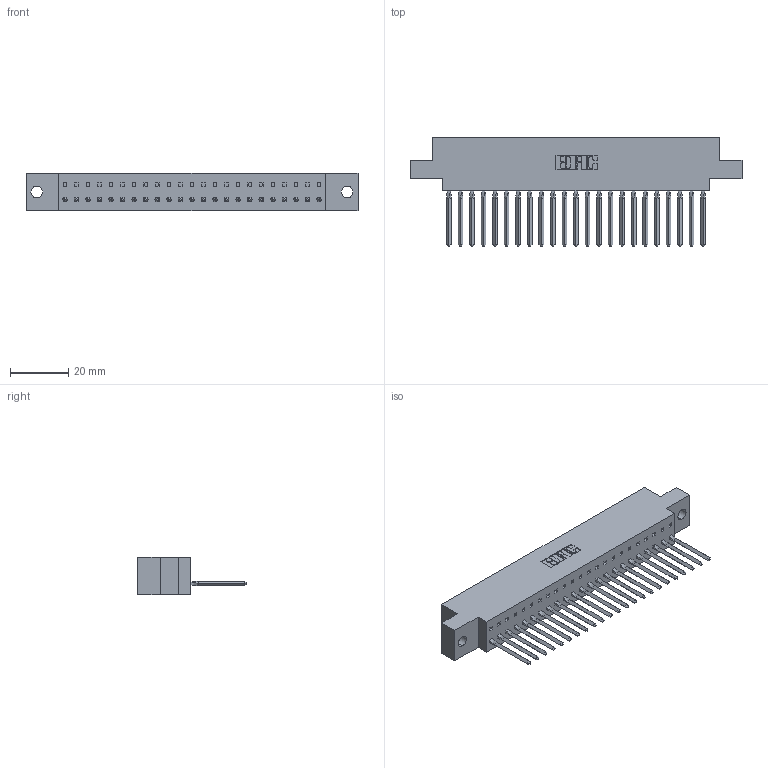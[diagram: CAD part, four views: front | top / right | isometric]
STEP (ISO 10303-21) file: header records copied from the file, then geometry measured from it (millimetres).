
FILE_DESCRIPTION (( 'STEP AP203' ), '1' );
FILE_NAME ('317-023-541-604.STEP', '2020-02-27T17:47:08', ( '' ), ( '' ), 'SwSTEP 2.0', 'SolidWorks 2016', '' );
FILE_SCHEMA (( 'CONFIG_CONTROL_DESIGN' ));
Length unit declared in the file: inch
Products named in the file (3): 317 Part_.156 Dia - TH; 317-290-002_541; 317-023-541-604
Assembly tree (24 placements, depth 2):
  317-023-541-604
    317 Part_.156 Dia - TH
    317-290-002_541  x23
Bounding box: 113.84 x 37.34 x 12.7 mm (x, y, z)
Volume: 17789.4 mm3; surface area: 24322.2 mm2
Topology: 24 solids, 24 shells, 3598 faces, 10257 edges, 6668 vertices
Faces by surface type: plane 2910, cylinder 596, bspline 92
Entity records: 36712 total; most frequent: CARTESIAN_POINT 7158, ORIENTED_EDGE 6434, DIRECTION 5271, EDGE_CURVE 3217, LINE 2853, VECTOR 2853, VERTEX_POINT 2136, AXIS2_PLACEMENT_3D 1209
